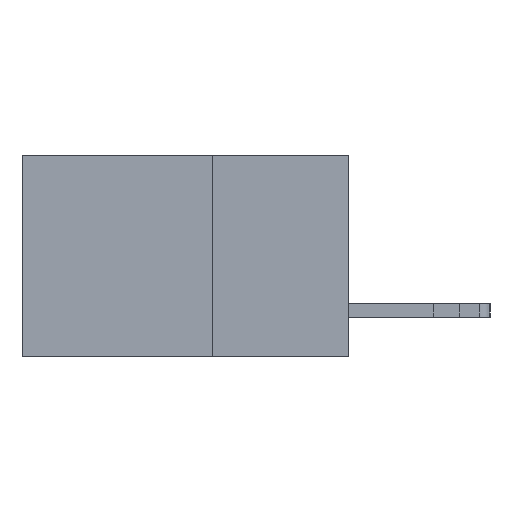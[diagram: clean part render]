
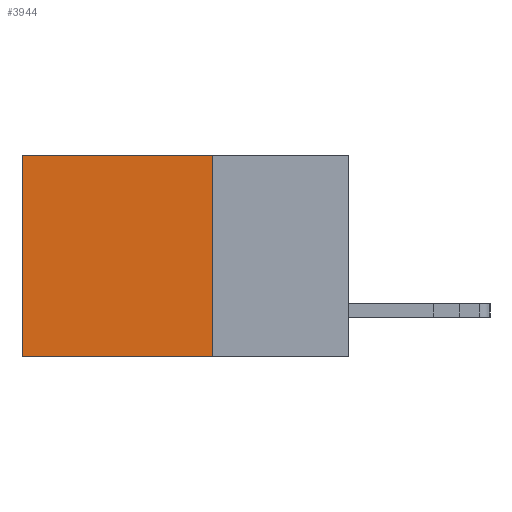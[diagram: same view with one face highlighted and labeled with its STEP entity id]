
A CAD part, left-side view. The second image highlights one B-rep face of the part: STEP entity #3944.
In plain terms, the highlighted planar face has unit normal (-1, 0, 0).
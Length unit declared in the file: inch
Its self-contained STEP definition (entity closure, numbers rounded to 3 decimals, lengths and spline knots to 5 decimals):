
#97 = DIRECTION ( 'NONE',  ( 0., 1., 0. ) ) ;
#275 = EDGE_CURVE ( 'NONE', #1695, #10461, #2306, .T. ) ;
#304 = VERTEX_POINT ( 'NONE', #9811 ) ;
#470 = DIRECTION ( 'NONE',  ( 1., 0., 0. ) ) ;
#844 = CARTESIAN_POINT ( 'NONE',  ( 0.298, 0.25, 0. ) ) ;
#951 = CARTESIAN_POINT ( 'NONE',  ( 0.298, 0.25, 0. ) ) ;
#1438 = EDGE_CURVE ( 'NONE', #5653, #10461, #9382, .T. ) ;
#1572 = LINE ( 'NONE', #9419, #9139 ) ;
#1695 = VERTEX_POINT ( 'NONE', #3671 ) ;
#2105 = CARTESIAN_POINT ( 'NONE',  ( 0.298, 0.6, 0. ) ) ;
#2251 = AXIS2_PLACEMENT_3D ( 'NONE', #844, #470, #8620 ) ;
#2306 = LINE ( 'NONE', #4213, #9564 ) ;
#2390 = DIRECTION ( 'NONE',  ( 0., 0., -1. ) ) ;
#3039 = CARTESIAN_POINT ( 'NONE',  ( 0.298, 0.6, 0. ) ) ;
#3671 = CARTESIAN_POINT ( 'NONE',  ( 0.298, 0.25, -0.37 ) ) ;
#3944 = ADVANCED_FACE ( 'NONE', ( #7904 ), #9140, .F. ) ;
#4213 = CARTESIAN_POINT ( 'NONE',  ( 0.298, 0.25, -0.37 ) ) ;
#5414 = ORIENTED_EDGE ( 'NONE', *, *, #6250, .T. ) ;
#5653 = VERTEX_POINT ( 'NONE', #3039 ) ;
#5670 = EDGE_LOOP ( 'NONE', ( #11435, #7528, #11923, #5414 ) ) ;
#5929 = DIRECTION ( 'NONE',  ( 0., 1., 0. ) ) ;
#6250 = EDGE_CURVE ( 'NONE', #304, #5653, #8841, .T. ) ;
#6534 = DIRECTION ( 'NONE',  ( 0., 0., -1. ) ) ;
#6646 = EDGE_CURVE ( 'NONE', #304, #1695, #1572, .T. ) ;
#7528 = ORIENTED_EDGE ( 'NONE', *, *, #275, .F. ) ;
#7904 = FACE_OUTER_BOUND ( 'NONE', #5670, .T. ) ;
#8620 = DIRECTION ( 'NONE',  ( 0., 0., -1. ) ) ;
#8841 = LINE ( 'NONE', #951, #11088 ) ;
#9063 = VECTOR ( 'NONE', #2390, 39.37008 ) ;
#9139 = VECTOR ( 'NONE', #6534, 39.37008 ) ;
#9140 = PLANE ( 'NONE',  #2251 ) ;
#9382 = LINE ( 'NONE', #2105, #9063 ) ;
#9419 = CARTESIAN_POINT ( 'NONE',  ( 0.298, 0.25, 0. ) ) ;
#9564 = VECTOR ( 'NONE', #97, 39.37008 ) ;
#9811 = CARTESIAN_POINT ( 'NONE',  ( 0.298, 0.25, 0. ) ) ;
#10461 = VERTEX_POINT ( 'NONE', #12655 ) ;
#11088 = VECTOR ( 'NONE', #5929, 39.37008 ) ;
#11435 = ORIENTED_EDGE ( 'NONE', *, *, #1438, .T. ) ;
#11923 = ORIENTED_EDGE ( 'NONE', *, *, #6646, .F. ) ;
#12655 = CARTESIAN_POINT ( 'NONE',  ( 0.298, 0.6, -0.37 ) ) ;
